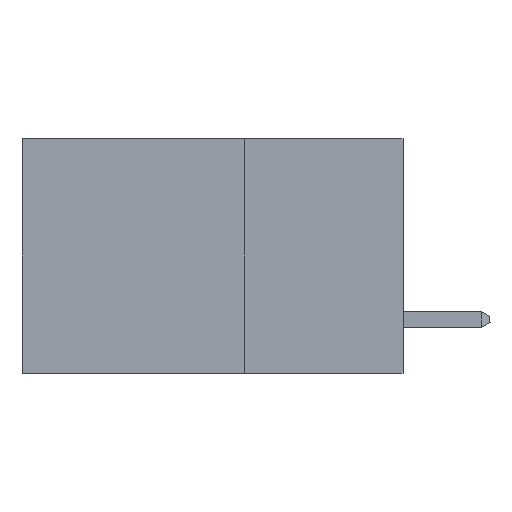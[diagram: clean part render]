
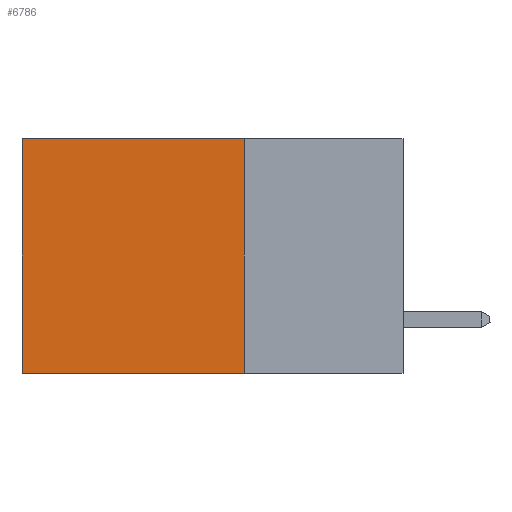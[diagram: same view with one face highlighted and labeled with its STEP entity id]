
A CAD part, left-side view. The second image highlights one B-rep face of the part: STEP entity #6786.
In plain terms, the highlighted planar face has unit normal (-1, 0, 0).
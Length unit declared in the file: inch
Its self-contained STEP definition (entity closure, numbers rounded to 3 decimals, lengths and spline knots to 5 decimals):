
#177 = CARTESIAN_POINT ( 'NONE',  ( 0.2875, 0.25, -0.37 ) ) ;
#1145 = CARTESIAN_POINT ( 'NONE',  ( 0.2875, 0.6, 0. ) ) ;
#1338 = EDGE_CURVE ( 'NONE', #2685, #8491, #9569, .T. ) ;
#1413 = LINE ( 'NONE', #177, #3669 ) ;
#1904 = ORIENTED_EDGE ( 'NONE', *, *, #9567, .F. ) ;
#2025 = PLANE ( 'NONE',  #13564 ) ;
#2685 = VERTEX_POINT ( 'NONE', #4123 ) ;
#2813 = FACE_OUTER_BOUND ( 'NONE', #14415, .T. ) ;
#2872 = LINE ( 'NONE', #5095, #9063 ) ;
#2887 = CARTESIAN_POINT ( 'NONE',  ( 0.2875, 0.25, -0.37 ) ) ;
#3099 = ORIENTED_EDGE ( 'NONE', *, *, #1338, .T. ) ;
#3227 = DIRECTION ( 'NONE',  ( 0., 0., -1. ) ) ;
#3492 = DIRECTION ( 'NONE',  ( 0., 0., -1. ) ) ;
#3669 = VECTOR ( 'NONE', #8635, 39.37008 ) ;
#4023 = EDGE_CURVE ( 'NONE', #12060, #11380, #1413, .T. ) ;
#4123 = CARTESIAN_POINT ( 'NONE',  ( 0.2875, 0.25, 0. ) ) ;
#4221 = CARTESIAN_POINT ( 'NONE',  ( 0.2875, 0.25, 0. ) ) ;
#5095 = CARTESIAN_POINT ( 'NONE',  ( 0.2875, 0.6, 0. ) ) ;
#6757 = DIRECTION ( 'NONE',  ( 1., 0., 0. ) ) ;
#6786 = ADVANCED_FACE ( 'NONE', ( #2813 ), #2025, .F. ) ;
#8491 = VERTEX_POINT ( 'NONE', #1145 ) ;
#8635 = DIRECTION ( 'NONE',  ( 0., 1., 0. ) ) ;
#8704 = DIRECTION ( 'NONE',  ( 0., 0., -1. ) ) ;
#9063 = VECTOR ( 'NONE', #8704, 39.37008 ) ;
#9567 = EDGE_CURVE ( 'NONE', #2685, #12060, #10279, .T. ) ;
#9569 = LINE ( 'NONE', #4221, #12380 ) ;
#10279 = LINE ( 'NONE', #10661, #11218 ) ;
#10661 = CARTESIAN_POINT ( 'NONE',  ( 0.2875, 0.25, 0. ) ) ;
#11218 = VECTOR ( 'NONE', #3492, 39.37008 ) ;
#11380 = VERTEX_POINT ( 'NONE', #15265 ) ;
#11517 = DIRECTION ( 'NONE',  ( 0., 1., 0. ) ) ;
#11724 = CARTESIAN_POINT ( 'NONE',  ( 0.2875, 0.25, 0. ) ) ;
#12060 = VERTEX_POINT ( 'NONE', #2887 ) ;
#12308 = ORIENTED_EDGE ( 'NONE', *, *, #12512, .T. ) ;
#12380 = VECTOR ( 'NONE', #11517, 39.37008 ) ;
#12512 = EDGE_CURVE ( 'NONE', #8491, #11380, #2872, .T. ) ;
#13564 = AXIS2_PLACEMENT_3D ( 'NONE', #11724, #6757, #3227 ) ;
#14040 = ORIENTED_EDGE ( 'NONE', *, *, #4023, .F. ) ;
#14415 = EDGE_LOOP ( 'NONE', ( #12308, #14040, #1904, #3099 ) ) ;
#15265 = CARTESIAN_POINT ( 'NONE',  ( 0.2875, 0.6, -0.37 ) ) ;
